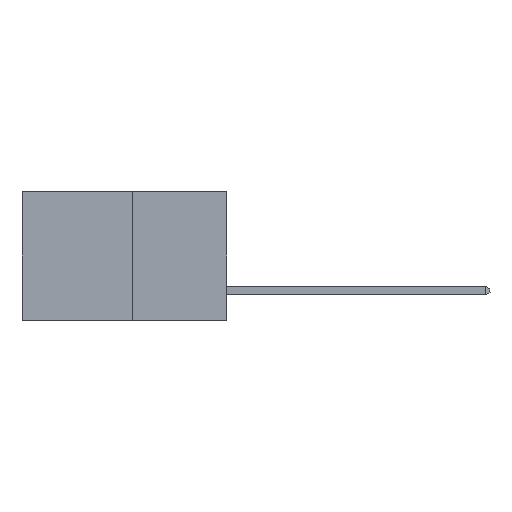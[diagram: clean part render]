
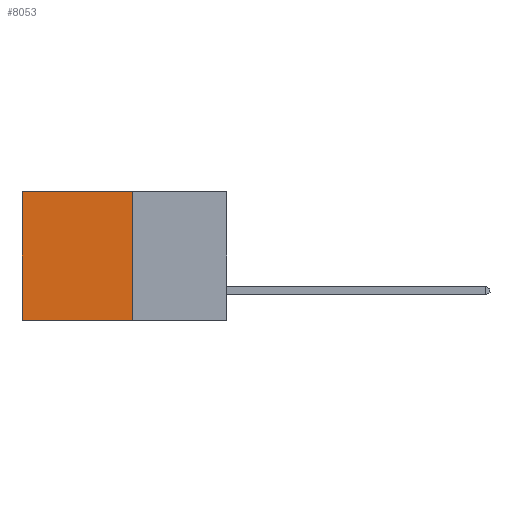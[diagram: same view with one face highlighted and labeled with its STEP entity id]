
A CAD part, left-side view. The second image highlights one B-rep face of the part: STEP entity #8053.
In plain terms, the highlighted planar face has unit normal (-1, 0, 0).
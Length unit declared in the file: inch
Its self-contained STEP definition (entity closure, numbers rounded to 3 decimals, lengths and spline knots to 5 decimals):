
#101 = ORIENTED_EDGE ( 'NONE', *, *, #7498, .T. ) ;
#317 = VERTEX_POINT ( 'NONE', #3959 ) ;
#328 = ORIENTED_EDGE ( 'NONE', *, *, #6179, .F. ) ;
#417 = CARTESIAN_POINT ( 'NONE',  ( 0.277, 0.59, -0.37 ) ) ;
#1435 = VECTOR ( 'NONE', #3214, 39.37008 ) ;
#2206 = ORIENTED_EDGE ( 'NONE', *, *, #4478, .T. ) ;
#2663 = VERTEX_POINT ( 'NONE', #417 ) ;
#2804 = VERTEX_POINT ( 'NONE', #4014 ) ;
#2999 = CARTESIAN_POINT ( 'NONE',  ( 0.277, 0.27, -0.37 ) ) ;
#3209 = ORIENTED_EDGE ( 'NONE', *, *, #6955, .F. ) ;
#3214 = DIRECTION ( 'NONE',  ( 0., 0., -1. ) ) ;
#3258 = CARTESIAN_POINT ( 'NONE',  ( 0.277, 0.59, -0.37 ) ) ;
#3452 = VECTOR ( 'NONE', #4757, 39.37008 ) ;
#3479 = VECTOR ( 'NONE', #8674, 39.37008 ) ;
#3695 = DIRECTION ( 'NONE',  ( 1., 0., 0. ) ) ;
#3959 = CARTESIAN_POINT ( 'NONE',  ( 0.277, 0.27, 0. ) ) ;
#3987 = EDGE_LOOP ( 'NONE', ( #2206, #328, #3209, #101 ) ) ;
#4014 = CARTESIAN_POINT ( 'NONE',  ( 0.277, 0.27, -0.37 ) ) ;
#4478 = EDGE_CURVE ( 'NONE', #8786, #2663, #8800, .T. ) ;
#4587 = CARTESIAN_POINT ( 'NONE',  ( 0.277, 0.59, 0. ) ) ;
#4588 = CARTESIAN_POINT ( 'NONE',  ( 0.277, 0.27, -0.37 ) ) ;
#4757 = DIRECTION ( 'NONE',  ( 0., 1., 0. ) ) ;
#6002 = VECTOR ( 'NONE', #7646, 39.37008 ) ;
#6179 = EDGE_CURVE ( 'NONE', #2804, #2663, #7216, .T. ) ;
#6873 = CARTESIAN_POINT ( 'NONE',  ( 0.277, 0.27, 0. ) ) ;
#6955 = EDGE_CURVE ( 'NONE', #317, #2804, #7843, .T. ) ;
#6977 = CARTESIAN_POINT ( 'NONE',  ( 0.277, 0.27, -0.37 ) ) ;
#7196 = LINE ( 'NONE', #6873, #3452 ) ;
#7216 = LINE ( 'NONE', #4588, #3479 ) ;
#7498 = EDGE_CURVE ( 'NONE', #317, #8786, #7196, .T. ) ;
#7646 = DIRECTION ( 'NONE',  ( 0., 0., -1. ) ) ;
#7843 = LINE ( 'NONE', #6977, #6002 ) ;
#7887 = PLANE ( 'NONE',  #8410 ) ;
#7970 = FACE_OUTER_BOUND ( 'NONE', #3987, .T. ) ;
#8053 = ADVANCED_FACE ( 'NONE', ( #7970 ), #7887, .F. ) ;
#8410 = AXIS2_PLACEMENT_3D ( 'NONE', #2999, #3695, #8545 ) ;
#8545 = DIRECTION ( 'NONE',  ( 0., 0., -1. ) ) ;
#8674 = DIRECTION ( 'NONE',  ( 0., 1., 0. ) ) ;
#8786 = VERTEX_POINT ( 'NONE', #4587 ) ;
#8800 = LINE ( 'NONE', #3258, #1435 ) ;
